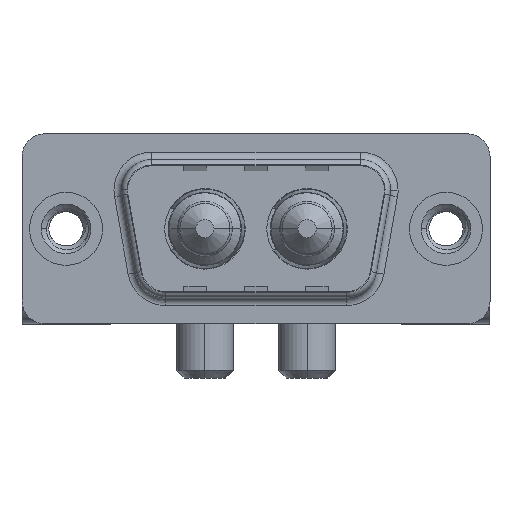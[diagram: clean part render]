
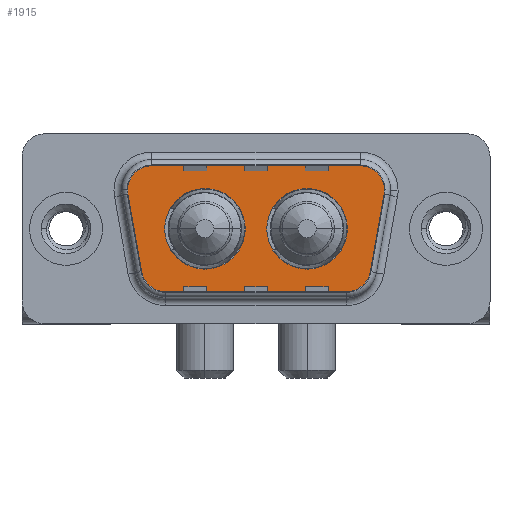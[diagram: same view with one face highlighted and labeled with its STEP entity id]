
A CAD part, top view. The second image highlights one B-rep face of the part: STEP entity #1915.
In plain terms, the highlighted planar face has unit normal (0, 0, 1).
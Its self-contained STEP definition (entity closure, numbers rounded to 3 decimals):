
#139 = EDGE_LOOP ( 'NONE', ( #11219, #2630 ) ) ;
#248 = AXIS2_PLACEMENT_3D ( 'NONE', #2237, #6046, #9905 ) ;
#350 = VERTEX_POINT ( 'NONE', #7516 ) ;
#374 = CARTESIAN_POINT ( 'NONE',  ( 18.51, 0., 0. ) ) ;
#376 = FACE_OUTER_BOUND ( 'NONE', #9836, .T. ) ;
#1157 = VERTEX_POINT ( 'NONE', #10223 ) ;
#1562 = FACE_BOUND ( 'NONE', #139, .T. ) ;
#1574 = CARTESIAN_POINT ( 'NONE',  ( 3.466, 2.553, 0. ) ) ;
#1605 = CARTESIAN_POINT ( 'NONE',  ( 19.564, 2.9, 0. ) ) ;
#1633 = CIRCLE ( 'NONE', #10746, 2.65 ) ;
#1636 = DIRECTION ( 'NONE',  ( 0.174, -0.985, 0. ) ) ;
#1765 = ORIENTED_EDGE ( 'NONE', *, *, #10626, .F. ) ;
#1860 = VERTEX_POINT ( 'NONE', #10121 ) ;
#1914 = CARTESIAN_POINT ( 'NONE',  ( 11.79, 0., 0. ) ) ;
#1915 = ADVANCED_FACE ( 'NONE', ( #1562, #3218, #376 ), #11959, .T. ) ;
#2106 = DIRECTION ( 'NONE',  ( -1., 0., 0. ) ) ;
#2177 = DIRECTION ( 'NONE',  ( 1., 0., 0. ) ) ;
#2237 = CARTESIAN_POINT ( 'NONE',  ( 18.541, -2.9, 0. ) ) ;
#2332 = DIRECTION ( 'NONE',  ( 1., 0., 0. ) ) ;
#2513 = DIRECTION ( 'NONE',  ( 1., 0., 0. ) ) ;
#2611 = VERTEX_POINT ( 'NONE', #1914 ) ;
#2630 = ORIENTED_EDGE ( 'NONE', *, *, #4755, .F. ) ;
#2646 = LINE ( 'NONE', #1574, #6423 ) ;
#2662 = CIRCLE ( 'NONE', #248, 2. ) ;
#2690 = DIRECTION ( 'NONE',  ( -1., 0., 0. ) ) ;
#2868 = DIRECTION ( 'NONE',  ( 0., 0., 1. ) ) ;
#2938 = ORIENTED_EDGE ( 'NONE', *, *, #5608, .T. ) ;
#3062 = CARTESIAN_POINT ( 'NONE',  ( 5.436, 2.9, 0. ) ) ;
#3120 = DIRECTION ( 'NONE',  ( 0., 0., 1. ) ) ;
#3137 = CARTESIAN_POINT ( 'NONE',  ( 9.14, 0., 0. ) ) ;
#3218 = FACE_BOUND ( 'NONE', #8071, .T. ) ;
#3283 = CARTESIAN_POINT ( 'NONE',  ( 18.541, -2.9, 0. ) ) ;
#3442 = ORIENTED_EDGE ( 'NONE', *, *, #6450, .T. ) ;
#3473 = CARTESIAN_POINT ( 'NONE',  ( 15.86, 0., 0. ) ) ;
#3631 = ORIENTED_EDGE ( 'NONE', *, *, #12485, .T. ) ;
#3665 = AXIS2_PLACEMENT_3D ( 'NONE', #5980, #5161, #2106 ) ;
#3782 = AXIS2_PLACEMENT_3D ( 'NONE', #3283, #7159, #2332 ) ;
#4036 = CARTESIAN_POINT ( 'NONE',  ( 21.564, 2.9, 0. ) ) ;
#4161 = DIRECTION ( 'NONE',  ( 1., 0., 0. ) ) ;
#4405 = VERTEX_POINT ( 'NONE', #10506 ) ;
#4542 = LINE ( 'NONE', #8397, #8314 ) ;
#4660 = VERTEX_POINT ( 'NONE', #10762 ) ;
#4755 = EDGE_CURVE ( 'NONE', #1860, #9238, #1633, .T. ) ;
#4838 = CARTESIAN_POINT ( 'NONE',  ( 15.86, 0., 0. ) ) ;
#4993 = CARTESIAN_POINT ( 'NONE',  ( 4.489, -3.247, 0. ) ) ;
#5069 = DIRECTION ( 'NONE',  ( 0.174, 0.985, 0. ) ) ;
#5102 = CIRCLE ( 'NONE', #3665, 2. ) ;
#5161 = DIRECTION ( 'NONE',  ( 0., 0., 1. ) ) ;
#5207 = AXIS2_PLACEMENT_3D ( 'NONE', #3137, #9723, #10928 ) ;
#5278 = ORIENTED_EDGE ( 'NONE', *, *, #6578, .T. ) ;
#5291 = VECTOR ( 'NONE', #2690, 1000. ) ;
#5402 = VERTEX_POINT ( 'NONE', #11911 ) ;
#5554 = LINE ( 'NONE', #9154, #5291 ) ;
#5608 = EDGE_CURVE ( 'NONE', #8909, #5402, #7094, .T. ) ;
#5724 = EDGE_CURVE ( 'NONE', #5728, #4660, #5554, .T. ) ;
#5728 = VERTEX_POINT ( 'NONE', #7339 ) ;
#5802 = EDGE_CURVE ( 'NONE', #8744, #4405, #4542, .T. ) ;
#5892 = DIRECTION ( 'NONE',  ( -1., 0., 0. ) ) ;
#5980 = CARTESIAN_POINT ( 'NONE',  ( 19.564, 2.9, 0. ) ) ;
#6010 = AXIS2_PLACEMENT_3D ( 'NONE', #9198, #11166, #4161 ) ;
#6046 = DIRECTION ( 'NONE',  ( 0., 0., 1. ) ) ;
#6316 = EDGE_CURVE ( 'NONE', #9238, #1860, #6909, .T. ) ;
#6409 = CIRCLE ( 'NONE', #5207, 2.65 ) ;
#6423 = VECTOR ( 'NONE', #1636, 1000. ) ;
#6435 = DIRECTION ( 'NONE',  ( 0., 0., 1. ) ) ;
#6450 = EDGE_CURVE ( 'NONE', #5402, #7372, #5102, .T. ) ;
#6509 = DIRECTION ( 'NONE',  ( 1., 0., 0. ) ) ;
#6578 = EDGE_CURVE ( 'NONE', #4660, #1157, #9522, .T. ) ;
#6592 = EDGE_CURVE ( 'NONE', #4405, #8909, #2662, .T. ) ;
#6803 = DIRECTION ( 'NONE',  ( 1., 0., 0. ) ) ;
#6909 = CIRCLE ( 'NONE', #7318, 2.65 ) ;
#7094 = LINE ( 'NONE', #8042, #8297 ) ;
#7159 = DIRECTION ( 'NONE',  ( 0., 0., 1. ) ) ;
#7222 = DIRECTION ( 'NONE',  ( 0., 0., 1. ) ) ;
#7318 = AXIS2_PLACEMENT_3D ( 'NONE', #4838, #2868, #6803 ) ;
#7339 = CARTESIAN_POINT ( 'NONE',  ( 19.564, 4.9, 0. ) ) ;
#7372 = VERTEX_POINT ( 'NONE', #4036 ) ;
#7516 = CARTESIAN_POINT ( 'NONE',  ( 6.49, 0., 0. ) ) ;
#7609 = CARTESIAN_POINT ( 'NONE',  ( 6.459, -2.9, 0. ) ) ;
#7875 = ORIENTED_EDGE ( 'NONE', *, *, #11965, .F. ) ;
#8042 = CARTESIAN_POINT ( 'NONE',  ( 21.534, 2.553, 0. ) ) ;
#8071 = EDGE_LOOP ( 'NONE', ( #7875, #1765 ) ) ;
#8297 = VECTOR ( 'NONE', #5069, 1000. ) ;
#8314 = VECTOR ( 'NONE', #6509, 1000. ) ;
#8397 = CARTESIAN_POINT ( 'NONE',  ( 6.459, -4.9, 0. ) ) ;
#8744 = VERTEX_POINT ( 'NONE', #12087 ) ;
#8846 = ORIENTED_EDGE ( 'NONE', *, *, #12113, .T. ) ;
#8909 = VERTEX_POINT ( 'NONE', #9484 ) ;
#9026 = AXIS2_PLACEMENT_3D ( 'NONE', #7609, #10454, #5892 ) ;
#9142 = DIRECTION ( 'NONE',  ( -1., 0., 0. ) ) ;
#9154 = CARTESIAN_POINT ( 'NONE',  ( 5.436, 4.9, 0. ) ) ;
#9198 = CARTESIAN_POINT ( 'NONE',  ( 9.14, 0., 0. ) ) ;
#9238 = VERTEX_POINT ( 'NONE', #374 ) ;
#9484 = CARTESIAN_POINT ( 'NONE',  ( 20.511, -3.247, 0. ) ) ;
#9522 = CIRCLE ( 'NONE', #11140, 2. ) ;
#9604 = ORIENTED_EDGE ( 'NONE', *, *, #9927, .T. ) ;
#9631 = AXIS2_PLACEMENT_3D ( 'NONE', #1605, #6435, #9142 ) ;
#9723 = DIRECTION ( 'NONE',  ( 0., 0., 1. ) ) ;
#9810 = CIRCLE ( 'NONE', #6010, 2.65 ) ;
#9836 = EDGE_LOOP ( 'NONE', ( #10511, #2938, #3442, #8846, #12410, #5278, #3631, #9604, #10018 ) ) ;
#9905 = DIRECTION ( 'NONE',  ( 1., 0., 0. ) ) ;
#9927 = EDGE_CURVE ( 'NONE', #12391, #8744, #11237, .T. ) ;
#10018 = ORIENTED_EDGE ( 'NONE', *, *, #5802, .T. ) ;
#10121 = CARTESIAN_POINT ( 'NONE',  ( 13.21, 0., 0. ) ) ;
#10223 = CARTESIAN_POINT ( 'NONE',  ( 3.466, 2.553, 0. ) ) ;
#10444 = CIRCLE ( 'NONE', #9631, 2. ) ;
#10454 = DIRECTION ( 'NONE',  ( 0., 0., 1. ) ) ;
#10506 = CARTESIAN_POINT ( 'NONE',  ( 18.541, -4.9, 0. ) ) ;
#10511 = ORIENTED_EDGE ( 'NONE', *, *, #6592, .T. ) ;
#10626 = EDGE_CURVE ( 'NONE', #350, #2611, #9810, .T. ) ;
#10746 = AXIS2_PLACEMENT_3D ( 'NONE', #3473, #7222, #2513 ) ;
#10762 = CARTESIAN_POINT ( 'NONE',  ( 5.436, 4.9, 0. ) ) ;
#10928 = DIRECTION ( 'NONE',  ( 1., 0., 0. ) ) ;
#11140 = AXIS2_PLACEMENT_3D ( 'NONE', #3062, #3120, #2177 ) ;
#11166 = DIRECTION ( 'NONE',  ( 0., 0., 1. ) ) ;
#11219 = ORIENTED_EDGE ( 'NONE', *, *, #6316, .F. ) ;
#11237 = CIRCLE ( 'NONE', #9026, 2. ) ;
#11911 = CARTESIAN_POINT ( 'NONE',  ( 21.534, 2.553, 0. ) ) ;
#11959 = PLANE ( 'NONE',  #3782 ) ;
#11965 = EDGE_CURVE ( 'NONE', #2611, #350, #6409, .T. ) ;
#12087 = CARTESIAN_POINT ( 'NONE',  ( 6.459, -4.9, 0. ) ) ;
#12113 = EDGE_CURVE ( 'NONE', #7372, #5728, #10444, .T. ) ;
#12391 = VERTEX_POINT ( 'NONE', #4993 ) ;
#12410 = ORIENTED_EDGE ( 'NONE', *, *, #5724, .T. ) ;
#12485 = EDGE_CURVE ( 'NONE', #1157, #12391, #2646, .T. ) ;
